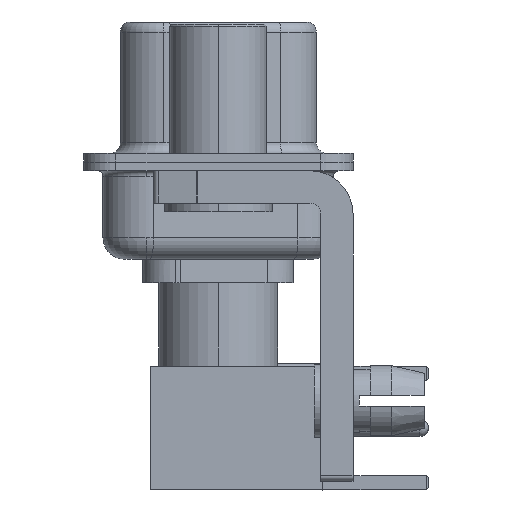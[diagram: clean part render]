
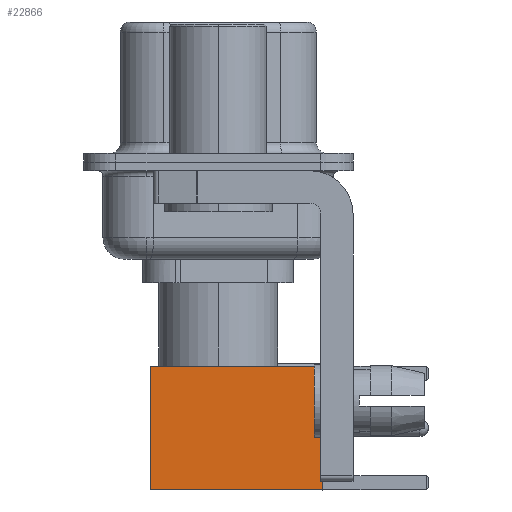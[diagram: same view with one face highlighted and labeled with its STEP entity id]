
A CAD part, left-side view. The second image highlights one B-rep face of the part: STEP entity #22866.
In plain terms, the highlighted face is planar.
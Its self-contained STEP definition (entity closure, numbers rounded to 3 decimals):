
#2315 = ORIENTED_EDGE ( 'NONE', *, *, #28143, .T. ) ;
#3559 = ORIENTED_EDGE ( 'NONE', *, *, #10014, .T. ) ;
#3669 = ORIENTED_EDGE ( 'NONE', *, *, #7372, .F. ) ;
#4193 = CARTESIAN_POINT ( 'NONE',  ( 0., 2.875, 0. ) ) ;
#4391 = DIRECTION ( 'NONE',  ( -1., 0., 0. ) ) ;
#4440 = CARTESIAN_POINT ( 'NONE',  ( -2.875, 2.875, 8. ) ) ;
#4852 = DIRECTION ( 'NONE',  ( -1., 0., 0. ) ) ;
#5436 = VECTOR ( 'NONE', #4852, 1000. ) ;
#6663 = VECTOR ( 'NONE', #18359, 1000. ) ;
#7372 = EDGE_CURVE ( 'NONE', #19368, #30425, #27260, .T. ) ;
#8080 = DIRECTION ( 'NONE',  ( 0., 1., 0. ) ) ;
#8236 = LINE ( 'NONE', #11040, #6663 ) ;
#8803 = VERTEX_POINT ( 'NONE', #9510 ) ;
#9510 = CARTESIAN_POINT ( 'NONE',  ( -2.875, 2.875, 0. ) ) ;
#10014 = EDGE_CURVE ( 'NONE', #19368, #24724, #8236, .T. ) ;
#11040 = CARTESIAN_POINT ( 'NONE',  ( 2.875, 2.875, 0. ) ) ;
#12570 = DIRECTION ( 'NONE',  ( 0., 0., -1. ) ) ;
#14280 = ORIENTED_EDGE ( 'NONE', *, *, #19366, .F. ) ;
#14762 = VECTOR ( 'NONE', #4391, 1000. ) ;
#18359 = DIRECTION ( 'NONE',  ( 0., 0., -1. ) ) ;
#19366 = EDGE_CURVE ( 'NONE', #30425, #8803, #27728, .T. ) ;
#19368 = VERTEX_POINT ( 'NONE', #22508 ) ;
#20668 = AXIS2_PLACEMENT_3D ( 'NONE', #22625, #8080, #27842 ) ;
#21274 = EDGE_LOOP ( 'NONE', ( #3559, #2315, #14280, #3669 ) ) ;
#21628 = CARTESIAN_POINT ( 'NONE',  ( 2.875, 2.875, 0. ) ) ;
#22508 = CARTESIAN_POINT ( 'NONE',  ( 2.875, 2.875, 8. ) ) ;
#22625 = CARTESIAN_POINT ( 'NONE',  ( 2.875, 2.875, 0. ) ) ;
#22866 = ADVANCED_FACE ( 'NONE', ( #30152 ), #30468, .T. ) ;
#24724 = VERTEX_POINT ( 'NONE', #21628 ) ;
#24774 = LINE ( 'NONE', #4193, #5436 ) ;
#25270 = CARTESIAN_POINT ( 'NONE',  ( -2.875, 2.875, 0. ) ) ;
#27260 = LINE ( 'NONE', #29561, #14762 ) ;
#27728 = LINE ( 'NONE', #25270, #28939 ) ;
#27842 = DIRECTION ( 'NONE',  ( 0., 0., 1. ) ) ;
#28143 = EDGE_CURVE ( 'NONE', #24724, #8803, #24774, .T. ) ;
#28939 = VECTOR ( 'NONE', #12570, 1000. ) ;
#29561 = CARTESIAN_POINT ( 'NONE',  ( 0., 2.875, 8. ) ) ;
#30152 = FACE_OUTER_BOUND ( 'NONE', #21274, .T. ) ;
#30425 = VERTEX_POINT ( 'NONE', #4440 ) ;
#30468 = PLANE ( 'NONE',  #20668 ) ;
